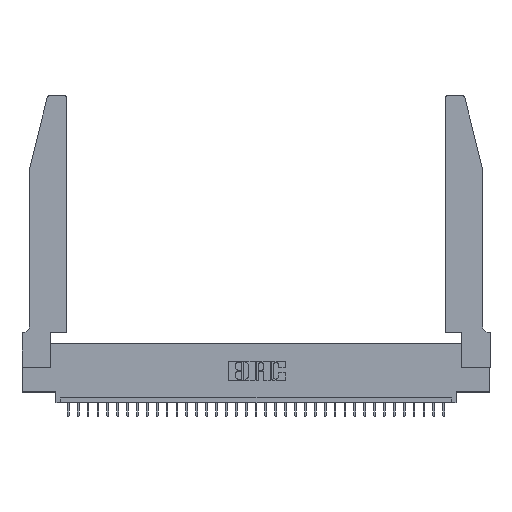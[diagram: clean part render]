
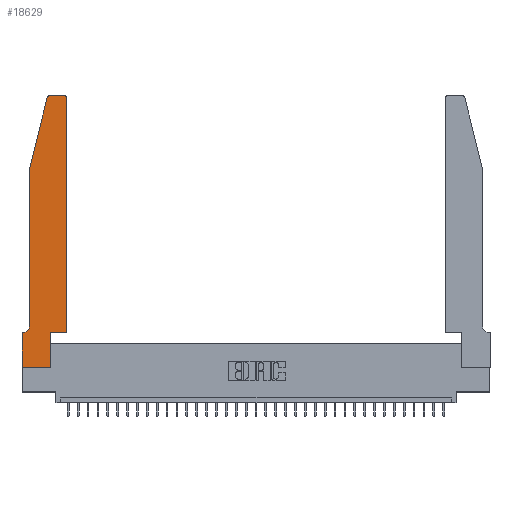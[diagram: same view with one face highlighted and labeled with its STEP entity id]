
A CAD part, top view. The second image highlights one B-rep face of the part: STEP entity #18629.
In plain terms, the highlighted planar face has unit normal (0, 0, 1).
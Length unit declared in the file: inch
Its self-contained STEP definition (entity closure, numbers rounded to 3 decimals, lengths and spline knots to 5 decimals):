
#839 = VERTEX_POINT ( 'NONE', #9632 ) ;
#1385 = CARTESIAN_POINT ( 'NONE',  ( 0.4505, 0.35, 0.37 ) ) ;
#1970 = DIRECTION ( 'NONE',  ( -1., 0., 0. ) ) ;
#2081 = PLANE ( 'NONE',  #32306 ) ;
#2467 = EDGE_CURVE ( 'NONE', #17954, #29422, #27906, .T. ) ;
#3295 = CARTESIAN_POINT ( 'NONE',  ( 0.4205, 2.75, 0.37 ) ) ;
#3334 = ORIENTED_EDGE ( 'NONE', *, *, #21417, .T. ) ;
#4535 = VECTOR ( 'NONE', #9752, 39.37008 ) ;
#4783 = CARTESIAN_POINT ( 'NONE',  ( 0.0755, 0.35, 0.37 ) ) ;
#4950 = CIRCLE ( 'NONE', #33546, 0.07 ) ;
#5416 = EDGE_CURVE ( 'NONE', #19760, #29506, #20818, .T. ) ;
#5671 = CARTESIAN_POINT ( 'NONE',  ( 0.0055, 0.42, 0.37 ) ) ;
#5909 = DIRECTION ( 'NONE',  ( 1., 0., 0. ) ) ;
#6413 = ORIENTED_EDGE ( 'NONE', *, *, #16398, .T. ) ;
#6813 = LINE ( 'NONE', #9612, #26204 ) ;
#6881 = VECTOR ( 'NONE', #12785, 39.37008 ) ;
#7591 = VERTEX_POINT ( 'NONE', #1385 ) ;
#8731 = LINE ( 'NONE', #33310, #11607 ) ;
#9261 = DIRECTION ( 'NONE',  ( 1., 0., 0. ) ) ;
#9612 = CARTESIAN_POINT ( 'NONE',  ( 0., 0., 0.37 ) ) ;
#9632 = CARTESIAN_POINT ( 'NONE',  ( 0., 0., 0.37 ) ) ;
#9670 = DIRECTION ( 'NONE',  ( 1., 0., 0. ) ) ;
#9752 = DIRECTION ( 'NONE',  ( 0., 1., 0. ) ) ;
#10208 = ORIENTED_EDGE ( 'NONE', *, *, #26535, .T. ) ;
#10659 = DIRECTION ( 'NONE',  ( 0., 0., 1. ) ) ;
#10953 = DIRECTION ( 'NONE',  ( 0., 0., -1. ) ) ;
#11224 = CARTESIAN_POINT ( 'NONE',  ( 0.2865, 0.35, 0.37 ) ) ;
#11228 = EDGE_CURVE ( 'NONE', #17050, #24261, #18291, .T. ) ;
#11487 = CARTESIAN_POINT ( 'NONE',  ( 0.4205, 2.72, 0.37 ) ) ;
#11607 = VECTOR ( 'NONE', #30192, 39.37008 ) ;
#11843 = ORIENTED_EDGE ( 'NONE', *, *, #2467, .T. ) ;
#11847 = AXIS2_PLACEMENT_3D ( 'NONE', #29999, #10659, #5909 ) ;
#11964 = EDGE_CURVE ( 'NONE', #7591, #30936, #23121, .T. ) ;
#12273 = CARTESIAN_POINT ( 'NONE',  ( 0.0755, 2., 0.37 ) ) ;
#12611 = VECTOR ( 'NONE', #31480, 39.37008 ) ;
#12785 = DIRECTION ( 'NONE',  ( 0., -1., 0. ) ) ;
#12973 = ORIENTED_EDGE ( 'NONE', *, *, #29750, .T. ) ;
#13149 = CARTESIAN_POINT ( 'NONE',  ( 0.0055, 0.35, 0.37 ) ) ;
#14694 = AXIS2_PLACEMENT_3D ( 'NONE', #11487, #30642, #17281 ) ;
#15174 = LINE ( 'NONE', #4783, #24912 ) ;
#15776 = LINE ( 'NONE', #20503, #6881 ) ;
#16398 = EDGE_CURVE ( 'NONE', #20734, #19453, #15174, .T. ) ;
#16566 = ORIENTED_EDGE ( 'NONE', *, *, #22860, .T. ) ;
#16806 = CARTESIAN_POINT ( 'NONE',  ( 0.4505, 2.72, 0.37 ) ) ;
#16841 = CARTESIAN_POINT ( 'NONE',  ( 0.0755, 2., 0.37 ) ) ;
#17050 = VERTEX_POINT ( 'NONE', #3295 ) ;
#17281 = DIRECTION ( 'NONE',  ( 1., 0., 0. ) ) ;
#17954 = VERTEX_POINT ( 'NONE', #30254 ) ;
#18247 = VECTOR ( 'NONE', #21177, 39.37008 ) ;
#18291 = LINE ( 'NONE', #31645, #12611 ) ;
#18629 = ADVANCED_FACE ( 'NONE', ( #26162 ), #2081, .T. ) ;
#19453 = VERTEX_POINT ( 'NONE', #34606 ) ;
#19760 = VERTEX_POINT ( 'NONE', #20175 ) ;
#19776 = EDGE_CURVE ( 'NONE', #19453, #839, #6813, .T. ) ;
#20175 = CARTESIAN_POINT ( 'NONE',  ( 0.2865, 0., 0.37 ) ) ;
#20298 = CIRCLE ( 'NONE', #14694, 0.03 ) ;
#20471 = EDGE_LOOP ( 'NONE', ( #34484, #10208, #11843, #12973, #16566, #6413, #27363, #3334, #29607, #28931, #21922, #22043 ) ) ;
#20503 = CARTESIAN_POINT ( 'NONE',  ( 0.0755, 2., 0.37 ) ) ;
#20734 = VERTEX_POINT ( 'NONE', #13149 ) ;
#20818 = LINE ( 'NONE', #23632, #18247 ) ;
#21177 = DIRECTION ( 'NONE',  ( 0., 1., 0. ) ) ;
#21417 = EDGE_CURVE ( 'NONE', #839, #19760, #33923, .T. ) ;
#21922 = ORIENTED_EDGE ( 'NONE', *, *, #11964, .T. ) ;
#22043 = ORIENTED_EDGE ( 'NONE', *, *, #27053, .T. ) ;
#22623 = CARTESIAN_POINT ( 'NONE',  ( 0., 0.35, 0.37 ) ) ;
#22860 = EDGE_CURVE ( 'NONE', #25850, #20734, #4950, .T. ) ;
#23121 = LINE ( 'NONE', #25597, #4535 ) ;
#23632 = CARTESIAN_POINT ( 'NONE',  ( 0.2865, 0.35, 0.37 ) ) ;
#24261 = VERTEX_POINT ( 'NONE', #25043 ) ;
#24912 = VECTOR ( 'NONE', #1970, 39.37008 ) ;
#25043 = CARTESIAN_POINT ( 'NONE',  ( 0.284, 2.75, 0.37 ) ) ;
#25597 = CARTESIAN_POINT ( 'NONE',  ( 0.4505, 0.35, 0.37 ) ) ;
#25803 = DIRECTION ( 'NONE',  ( -0.239, -0.971, 0. ) ) ;
#25850 = VERTEX_POINT ( 'NONE', #27989 ) ;
#25991 = DIRECTION ( 'NONE',  ( 0., -1., 0. ) ) ;
#26162 = FACE_OUTER_BOUND ( 'NONE', #20471, .T. ) ;
#26204 = VECTOR ( 'NONE', #25991, 39.37008 ) ;
#26222 = CARTESIAN_POINT ( 'NONE',  ( 0., 0., 0.37 ) ) ;
#26535 = EDGE_CURVE ( 'NONE', #24261, #17954, #29263, .T. ) ;
#27053 = EDGE_CURVE ( 'NONE', #30936, #17050, #20298, .T. ) ;
#27363 = ORIENTED_EDGE ( 'NONE', *, *, #19776, .T. ) ;
#27906 = LINE ( 'NONE', #12273, #29907 ) ;
#27989 = CARTESIAN_POINT ( 'NONE',  ( 0.0755, 0.42, 0.37 ) ) ;
#28931 = ORIENTED_EDGE ( 'NONE', *, *, #34598, .T. ) ;
#29263 = CIRCLE ( 'NONE', #11847, 0.03 ) ;
#29422 = VERTEX_POINT ( 'NONE', #16841 ) ;
#29506 = VERTEX_POINT ( 'NONE', #11224 ) ;
#29607 = ORIENTED_EDGE ( 'NONE', *, *, #5416, .T. ) ;
#29750 = EDGE_CURVE ( 'NONE', #29422, #25850, #15776, .T. ) ;
#29907 = VECTOR ( 'NONE', #25803, 39.37008 ) ;
#29999 = CARTESIAN_POINT ( 'NONE',  ( 0.284, 2.72, 0.37 ) ) ;
#30192 = DIRECTION ( 'NONE',  ( 1., 0., 0. ) ) ;
#30254 = CARTESIAN_POINT ( 'NONE',  ( 0.25487, 2.72718, 0.37 ) ) ;
#30642 = DIRECTION ( 'NONE',  ( 0., 0., 1. ) ) ;
#30936 = VERTEX_POINT ( 'NONE', #16806 ) ;
#31480 = DIRECTION ( 'NONE',  ( -1., 0., 0. ) ) ;
#31645 = CARTESIAN_POINT ( 'NONE',  ( 0.2605, 2.75, 0.37 ) ) ;
#32207 = DIRECTION ( 'NONE',  ( -1., 0., 0. ) ) ;
#32306 = AXIS2_PLACEMENT_3D ( 'NONE', #22623, #33333, #9261 ) ;
#32353 = VECTOR ( 'NONE', #9670, 39.37008 ) ;
#33310 = CARTESIAN_POINT ( 'NONE',  ( 0.4505, 0.35, 0.37 ) ) ;
#33333 = DIRECTION ( 'NONE',  ( 0., 0., 1. ) ) ;
#33546 = AXIS2_PLACEMENT_3D ( 'NONE', #5671, #10953, #32207 ) ;
#33923 = LINE ( 'NONE', #26222, #32353 ) ;
#34484 = ORIENTED_EDGE ( 'NONE', *, *, #11228, .T. ) ;
#34598 = EDGE_CURVE ( 'NONE', #29506, #7591, #8731, .T. ) ;
#34606 = CARTESIAN_POINT ( 'NONE',  ( 0., 0.35, 0.37 ) ) ;
